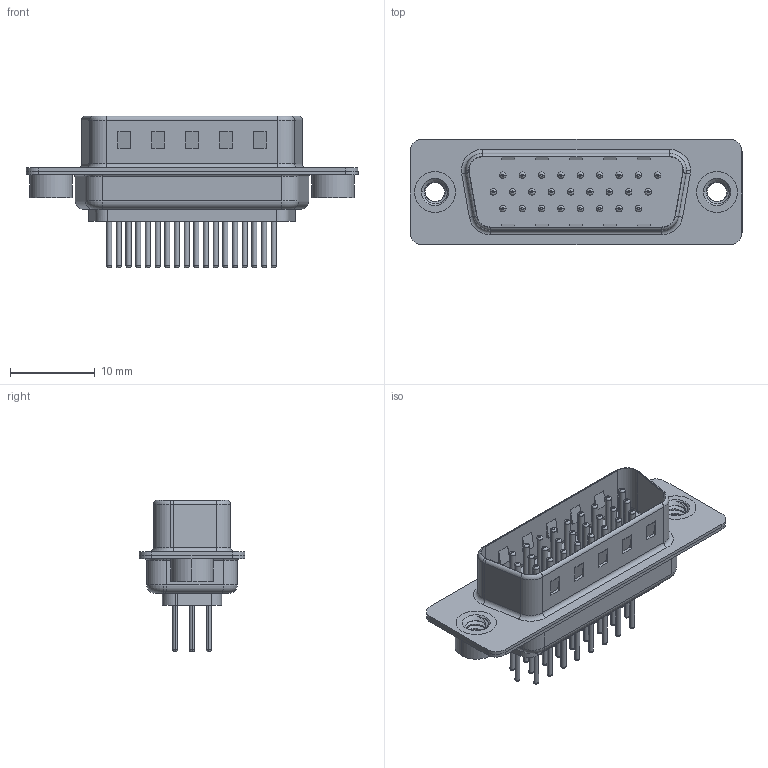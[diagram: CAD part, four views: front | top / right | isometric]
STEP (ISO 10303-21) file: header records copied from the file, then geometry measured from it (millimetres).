
FILE_DESCRIPTION (( 'STEP AP203' ), '1' );
FILE_NAME ('637-M26-330-BN2.STEP', '2018-11-19T23:36:27', ( '' ), ( '' ), 'SwSTEP 2.0', 'SolidWorks 2016', '' );
FILE_SCHEMA (( 'CONFIG_CONTROL_DESIGN' ));
Length unit declared in the file: millimetre
Products named in the file (8): 637M Shell Rear_26 Contacts; 637M Contact Row 1_30; 637M Contact Row 2_30; 637M Contact Row 3_30; 637M 4-40 Threaded Rivet; 637-M26-330-BN2; 637M Housing_26 Contacts; 637M Shell Front_26 Contacts
Assembly tree (31 placements, depth 2):
  637-M26-330-BN2
    637M Housing_26 Contacts
    637M Shell Front_26 Contacts
    637M Shell Rear_26 Contacts
    637M Contact Row 1_30  x9
    637M Contact Row 2_30  x9
    637M Contact Row 3_30  x8
    637M 4-40 Threaded Rivet  x2
Bounding box: 39.2 x 12.5 x 17.9 mm (x, y, z)
Volume: 1909.1 mm3; surface area: 5750.9 mm2
Topology: 31 solids, 31 shells, 1302 faces, 2781 edges, 1682 vertices
Faces by surface type: cylinder 497, torus 466, plane 321, cone 12, bspline 6
Entity records: 20597 total; most frequent: CARTESIAN_POINT 4478, DIRECTION 3368, ORIENTED_EDGE 2824, EDGE_CURVE 1412, AXIS2_PLACEMENT_3D 1370, VERTEX_POINT 894, EDGE_LOOP 758, CIRCLE 737
